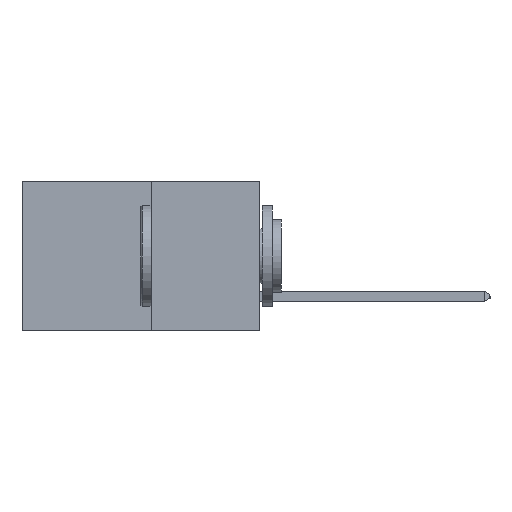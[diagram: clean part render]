
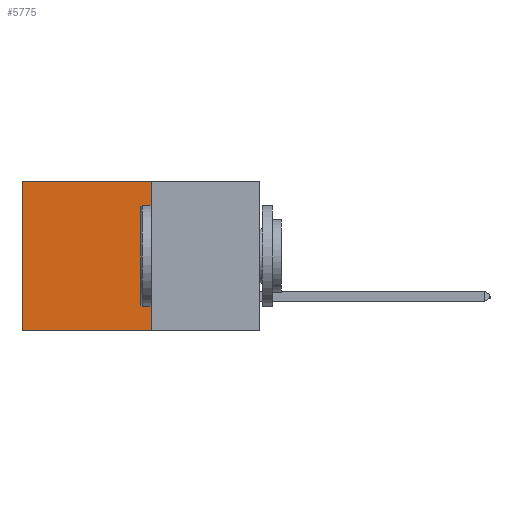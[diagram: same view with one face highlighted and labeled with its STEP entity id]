
A CAD part, left-side view. The second image highlights one B-rep face of the part: STEP entity #5775.
In plain terms, the highlighted planar face has unit normal (-1, 0, 0).
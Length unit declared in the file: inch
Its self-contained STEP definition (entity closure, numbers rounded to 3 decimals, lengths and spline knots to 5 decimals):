
#136 = ORIENTED_EDGE ( 'NONE', *, *, #9820, .T. ) ;
#1067 = VECTOR ( 'NONE', #1930, 39.37008 ) ;
#1523 = VERTEX_POINT ( 'NONE', #6748 ) ;
#1551 = VECTOR ( 'NONE', #10929, 39.37008 ) ;
#1653 = CARTESIAN_POINT ( 'NONE',  ( 0.277, 0.27, -0.37 ) ) ;
#1785 = VECTOR ( 'NONE', #7383, 39.37008 ) ;
#1905 = VERTEX_POINT ( 'NONE', #5932 ) ;
#1930 = DIRECTION ( 'NONE',  ( 0., 1., 0. ) ) ;
#1980 = CARTESIAN_POINT ( 'NONE',  ( 0.277, 0.27, -0.37 ) ) ;
#1984 = DIRECTION ( 'NONE',  ( 0., 0., -1. ) ) ;
#2160 = CARTESIAN_POINT ( 'NONE',  ( 0.277, 0.27, 0. ) ) ;
#2279 = ORIENTED_EDGE ( 'NONE', *, *, #6941, .F. ) ;
#2942 = EDGE_LOOP ( 'NONE', ( #7486, #5389, #2279, #136 ) ) ;
#4560 = EDGE_CURVE ( 'NONE', #6380, #12044, #10573, .T. ) ;
#5389 = ORIENTED_EDGE ( 'NONE', *, *, #6965, .F. ) ;
#5775 = ADVANCED_FACE ( 'NONE', ( #5956 ), #12735, .F. ) ;
#5932 = CARTESIAN_POINT ( 'NONE',  ( 0.277, 0.27, 0. ) ) ;
#5956 = FACE_OUTER_BOUND ( 'NONE', #2942, .T. ) ;
#6380 = VERTEX_POINT ( 'NONE', #7242 ) ;
#6748 = CARTESIAN_POINT ( 'NONE',  ( 0.277, 0.27, -0.37 ) ) ;
#6941 = EDGE_CURVE ( 'NONE', #1905, #1523, #13052, .T. ) ;
#6965 = EDGE_CURVE ( 'NONE', #1523, #12044, #9946, .T. ) ;
#7081 = CARTESIAN_POINT ( 'NONE',  ( 0.277, 0.59, -0.37 ) ) ;
#7242 = CARTESIAN_POINT ( 'NONE',  ( 0.277, 0.59, 0. ) ) ;
#7379 = VECTOR ( 'NONE', #1984, 39.37008 ) ;
#7383 = DIRECTION ( 'NONE',  ( 0., 0., -1. ) ) ;
#7459 = LINE ( 'NONE', #2160, #1551 ) ;
#7469 = CARTESIAN_POINT ( 'NONE',  ( 0.277, 0.59, -0.37 ) ) ;
#7486 = ORIENTED_EDGE ( 'NONE', *, *, #4560, .T. ) ;
#7532 = AXIS2_PLACEMENT_3D ( 'NONE', #12711, #12655, #12627 ) ;
#9820 = EDGE_CURVE ( 'NONE', #1905, #6380, #7459, .T. ) ;
#9946 = LINE ( 'NONE', #1653, #1067 ) ;
#10573 = LINE ( 'NONE', #7469, #1785 ) ;
#10929 = DIRECTION ( 'NONE',  ( 0., 1., 0. ) ) ;
#12044 = VERTEX_POINT ( 'NONE', #7081 ) ;
#12627 = DIRECTION ( 'NONE',  ( 0., 0., -1. ) ) ;
#12655 = DIRECTION ( 'NONE',  ( 1., 0., 0. ) ) ;
#12711 = CARTESIAN_POINT ( 'NONE',  ( 0.277, 0.27, -0.37 ) ) ;
#12735 = PLANE ( 'NONE',  #7532 ) ;
#13052 = LINE ( 'NONE', #1980, #7379 ) ;
